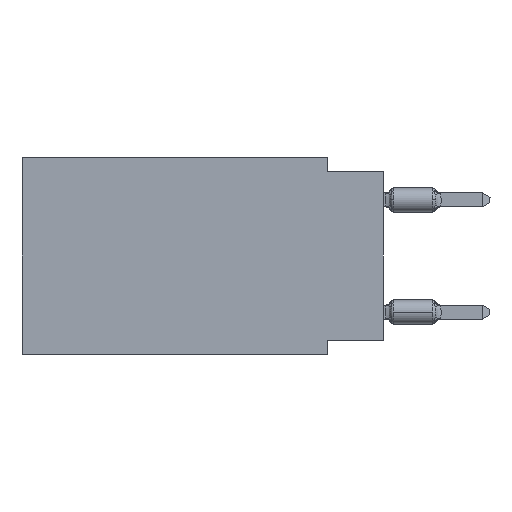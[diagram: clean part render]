
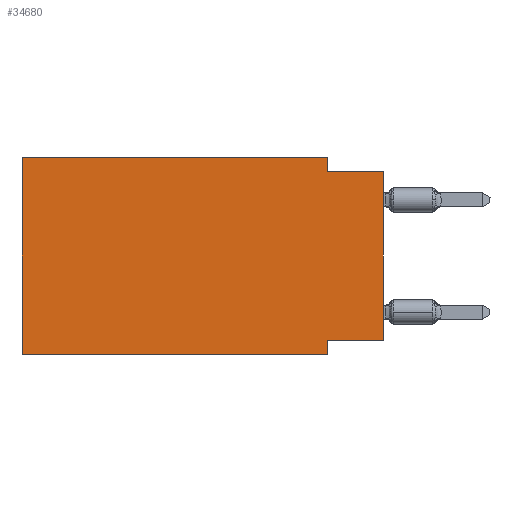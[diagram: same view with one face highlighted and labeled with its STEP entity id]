
A CAD part, left-side view. The second image highlights one B-rep face of the part: STEP entity #34680.
In plain terms, the highlighted planar face has unit normal (-1, 0, 0).
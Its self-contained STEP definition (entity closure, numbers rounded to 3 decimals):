
#656 = EDGE_CURVE ( 'NONE', #34385, #41192, #37328, .T. ) ;
#1357 = LINE ( 'NONE', #30664, #35772 ) ;
#1624 = CARTESIAN_POINT ( 'NONE',  ( 0., 2.54, 0. ) ) ;
#1867 = LINE ( 'NONE', #1624, #15129 ) ;
#1945 = EDGE_LOOP ( 'NONE', ( #13400, #25074, #12038, #16660, #40249, #9031, #15480, #16647 ) ) ;
#2116 = CARTESIAN_POINT ( 'NONE',  ( 0., 0., -0.635 ) ) ;
#6297 = CARTESIAN_POINT ( 'NONE',  ( 0., 2.54, -8.89 ) ) ;
#7540 = CARTESIAN_POINT ( 'NONE',  ( 0., 16.383, 0. ) ) ;
#7941 = CARTESIAN_POINT ( 'NONE',  ( 0., 16.383, -8.89 ) ) ;
#9031 = ORIENTED_EDGE ( 'NONE', *, *, #41527, .T. ) ;
#11250 = VECTOR ( 'NONE', #41354, 1000. ) ;
#12038 = ORIENTED_EDGE ( 'NONE', *, *, #22912, .F. ) ;
#13400 = ORIENTED_EDGE ( 'NONE', *, *, #37264, .T. ) ;
#14041 = VECTOR ( 'NONE', #37024, 1000. ) ;
#15129 = VECTOR ( 'NONE', #28703, 1000. ) ;
#15264 = CARTESIAN_POINT ( 'NONE',  ( 0., 16.383, 0. ) ) ;
#15480 = ORIENTED_EDGE ( 'NONE', *, *, #26251, .F. ) ;
#15762 = VECTOR ( 'NONE', #24695, 1000. ) ;
#16539 = VECTOR ( 'NONE', #28625, 1000. ) ;
#16647 = ORIENTED_EDGE ( 'NONE', *, *, #22348, .F. ) ;
#16660 = ORIENTED_EDGE ( 'NONE', *, *, #21681, .F. ) ;
#17873 = VERTEX_POINT ( 'NONE', #41572 ) ;
#17993 = VECTOR ( 'NONE', #42244, 1000. ) ;
#18077 = DIRECTION ( 'NONE',  ( 0., 0., 1. ) ) ;
#19653 = LINE ( 'NONE', #23727, #17993 ) ;
#20723 = AXIS2_PLACEMENT_3D ( 'NONE', #15264, #44606, #26561 ) ;
#21681 = EDGE_CURVE ( 'NONE', #41192, #40275, #1357, .T. ) ;
#22348 = EDGE_CURVE ( 'NONE', #31810, #44395, #37292, .T. ) ;
#22474 = PLANE ( 'NONE',  #20723 ) ;
#22912 = EDGE_CURVE ( 'NONE', #40275, #35656, #1867, .T. ) ;
#23043 = LINE ( 'NONE', #7941, #14041 ) ;
#23225 = CARTESIAN_POINT ( 'NONE',  ( 0., 2.54, -8.255 ) ) ;
#23727 = CARTESIAN_POINT ( 'NONE',  ( 0., 0., 0. ) ) ;
#24695 = DIRECTION ( 'NONE',  ( 0., -1., 0. ) ) ;
#25074 = ORIENTED_EDGE ( 'NONE', *, *, #25299, .F. ) ;
#25299 = EDGE_CURVE ( 'NONE', #35656, #17873, #42255, .T. ) ;
#26251 = EDGE_CURVE ( 'NONE', #44395, #36404, #42350, .T. ) ;
#26561 = DIRECTION ( 'NONE',  ( 0., 0., -1. ) ) ;
#27233 = CARTESIAN_POINT ( 'NONE',  ( 0., 2.54, -8.89 ) ) ;
#28056 = CARTESIAN_POINT ( 'NONE',  ( 0., 2.54, -0.635 ) ) ;
#28625 = DIRECTION ( 'NONE',  ( 0., 0., -1. ) ) ;
#28703 = DIRECTION ( 'NONE',  ( 0., 0., -1. ) ) ;
#30664 = CARTESIAN_POINT ( 'NONE',  ( 0., 16.383, 0. ) ) ;
#31003 = CARTESIAN_POINT ( 'NONE',  ( 0., 0., -8.255 ) ) ;
#31810 = VERTEX_POINT ( 'NONE', #42549 ) ;
#34385 = VERTEX_POINT ( 'NONE', #42941 ) ;
#34680 = ADVANCED_FACE ( 'NONE', ( #44370 ), #22474, .F. ) ;
#35656 = VERTEX_POINT ( 'NONE', #28056 ) ;
#35772 = VECTOR ( 'NONE', #45336, 1000. ) ;
#36404 = VERTEX_POINT ( 'NONE', #27233 ) ;
#37024 = DIRECTION ( 'NONE',  ( 0., -1., 0. ) ) ;
#37264 = EDGE_CURVE ( 'NONE', #31810, #17873, #19653, .T. ) ;
#37292 = LINE ( 'NONE', #31003, #11250 ) ;
#37328 = LINE ( 'NONE', #40205, #42061 ) ;
#40205 = CARTESIAN_POINT ( 'NONE',  ( 0., 16.383, 0. ) ) ;
#40249 = ORIENTED_EDGE ( 'NONE', *, *, #656, .F. ) ;
#40275 = VERTEX_POINT ( 'NONE', #46838 ) ;
#41192 = VERTEX_POINT ( 'NONE', #7540 ) ;
#41354 = DIRECTION ( 'NONE',  ( 0., 1., 0. ) ) ;
#41527 = EDGE_CURVE ( 'NONE', #34385, #36404, #23043, .T. ) ;
#41572 = CARTESIAN_POINT ( 'NONE',  ( 0., 0., -0.635 ) ) ;
#42061 = VECTOR ( 'NONE', #18077, 1000. ) ;
#42244 = DIRECTION ( 'NONE',  ( 0., 0., 1. ) ) ;
#42255 = LINE ( 'NONE', #2116, #15762 ) ;
#42350 = LINE ( 'NONE', #6297, #16539 ) ;
#42549 = CARTESIAN_POINT ( 'NONE',  ( 0., 0., -8.255 ) ) ;
#42941 = CARTESIAN_POINT ( 'NONE',  ( 0., 16.383, -8.89 ) ) ;
#44370 = FACE_OUTER_BOUND ( 'NONE', #1945, .T. ) ;
#44395 = VERTEX_POINT ( 'NONE', #23225 ) ;
#44606 = DIRECTION ( 'NONE',  ( 1., 0., 0. ) ) ;
#45336 = DIRECTION ( 'NONE',  ( 0., -1., 0. ) ) ;
#46838 = CARTESIAN_POINT ( 'NONE',  ( 0., 2.54, 0. ) ) ;
